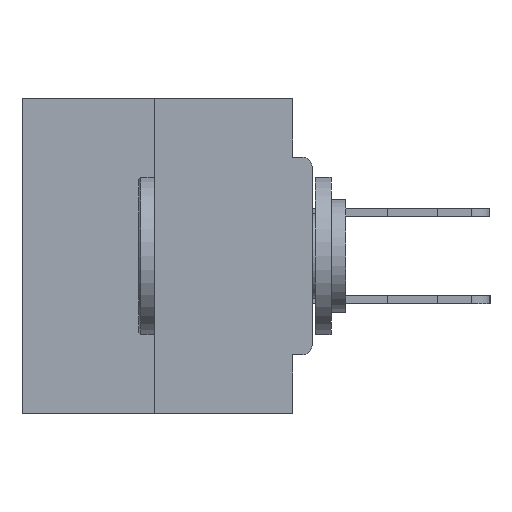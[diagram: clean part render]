
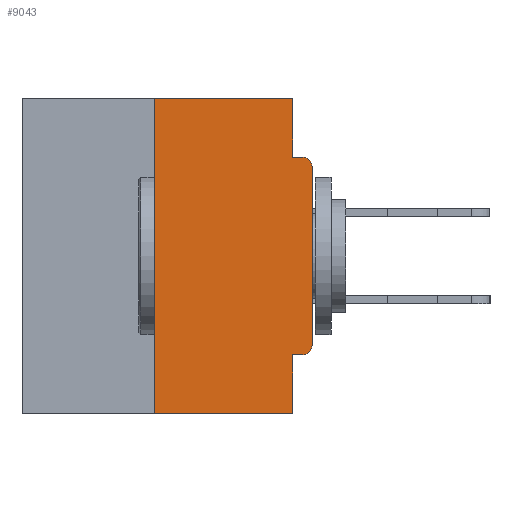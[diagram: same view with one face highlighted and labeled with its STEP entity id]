
A CAD part, left-side view. The second image highlights one B-rep face of the part: STEP entity #9043.
In plain terms, the highlighted planar face has unit normal (-1, 0, 0).
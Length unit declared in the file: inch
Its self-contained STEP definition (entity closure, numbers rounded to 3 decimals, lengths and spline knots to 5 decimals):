
#527 = CARTESIAN_POINT ( 'NONE',  ( 0., 0., -0.0935 ) ) ;
#830 = VECTOR ( 'NONE', #32874, 39.37008 ) ;
#1498 = CARTESIAN_POINT ( 'NONE',  ( 0., 0., 0. ) ) ;
#2949 = LINE ( 'NONE', #16704, #18603 ) ;
#3175 = LINE ( 'NONE', #33150, #6227 ) ;
#3206 = ORIENTED_EDGE ( 'NONE', *, *, #18143, .T. ) ;
#3600 = EDGE_CURVE ( 'NONE', #32147, #38464, #3175, .T. ) ;
#3841 = VERTEX_POINT ( 'NONE', #30647 ) ;
#5326 = LINE ( 'NONE', #1498, #29543 ) ;
#6178 = EDGE_CURVE ( 'NONE', #37746, #3841, #2949, .T. ) ;
#6227 = VECTOR ( 'NONE', #13628, 39.37008 ) ;
#6425 = CARTESIAN_POINT ( 'NONE',  ( 0., 0.25, 0. ) ) ;
#6603 = ORIENTED_EDGE ( 'NONE', *, *, #18887, .T. ) ;
#6707 = VECTOR ( 'NONE', #35863, 39.37008 ) ;
#7351 = DIRECTION ( 'NONE',  ( 0., 1., 0. ) ) ;
#9043 = ADVANCED_FACE ( 'NONE', ( #31865 ), #21742, .F. ) ;
#9212 = DIRECTION ( 'NONE',  ( -1., 0., 0. ) ) ;
#9318 = VERTEX_POINT ( 'NONE', #10560 ) ;
#9726 = CARTESIAN_POINT ( 'NONE',  ( 0., 0.031, 0. ) ) ;
#10375 = VERTEX_POINT ( 'NONE', #37322 ) ;
#10560 = CARTESIAN_POINT ( 'NONE',  ( 0., 0.015, -0.0935 ) ) ;
#11469 = AXIS2_PLACEMENT_3D ( 'NONE', #24979, #12421, #31970 ) ;
#12241 = EDGE_CURVE ( 'NONE', #3841, #30414, #36636, .T. ) ;
#12421 = DIRECTION ( 'NONE',  ( 1., 0., 0. ) ) ;
#12734 = CARTESIAN_POINT ( 'NONE',  ( 0., 0.031, -0.5 ) ) ;
#12976 = EDGE_CURVE ( 'NONE', #32429, #32147, #39574, .T. ) ;
#13628 = DIRECTION ( 'NONE',  ( 0., -1., 0. ) ) ;
#14148 = CIRCLE ( 'NONE', #14466, 0.015 ) ;
#14466 = AXIS2_PLACEMENT_3D ( 'NONE', #25701, #9212, #18907 ) ;
#14702 = CARTESIAN_POINT ( 'NONE',  ( 0., 0.25, 0. ) ) ;
#15215 = CIRCLE ( 'NONE', #40573, 0.015 ) ;
#16526 = DIRECTION ( 'NONE',  ( 0., -1., 0. ) ) ;
#16704 = CARTESIAN_POINT ( 'NONE',  ( 0., 0., -0.4065 ) ) ;
#17933 = VECTOR ( 'NONE', #29307, 39.37008 ) ;
#18143 = EDGE_CURVE ( 'NONE', #37746, #10375, #15215, .T. ) ;
#18603 = VECTOR ( 'NONE', #7351, 39.37008 ) ;
#18887 = EDGE_CURVE ( 'NONE', #32446, #9318, #14148, .T. ) ;
#18907 = DIRECTION ( 'NONE',  ( 0., 0., -1. ) ) ;
#18937 = ORIENTED_EDGE ( 'NONE', *, *, #34356, .T. ) ;
#19187 = ORIENTED_EDGE ( 'NONE', *, *, #12976, .F. ) ;
#19245 = DIRECTION ( 'NONE',  ( 0., 0., 1. ) ) ;
#19813 = VERTEX_POINT ( 'NONE', #25471 ) ;
#20963 = DIRECTION ( 'NONE',  ( 0., 0., 1. ) ) ;
#21742 = PLANE ( 'NONE',  #11469 ) ;
#21931 = ORIENTED_EDGE ( 'NONE', *, *, #32604, .T. ) ;
#22464 = EDGE_LOOP ( 'NONE', ( #37503, #19187, #18937, #27968, #35014, #3206, #21931, #6603, #24981, #36071 ) ) ;
#23118 = CARTESIAN_POINT ( 'NONE',  ( 0., 0.25, -0.5 ) ) ;
#24979 = CARTESIAN_POINT ( 'NONE',  ( 0., 0.46, 0. ) ) ;
#24981 = ORIENTED_EDGE ( 'NONE', *, *, #39985, .F. ) ;
#25471 = CARTESIAN_POINT ( 'NONE',  ( 0., 0.031, -0.0935 ) ) ;
#25658 = DIRECTION ( 'NONE',  ( 0., 0., -1. ) ) ;
#25701 = CARTESIAN_POINT ( 'NONE',  ( 0., 0.015, -0.1085 ) ) ;
#26360 = CARTESIAN_POINT ( 'NONE',  ( 0., 0., -0.1085 ) ) ;
#27088 = CARTESIAN_POINT ( 'NONE',  ( 0., 0.031, 0. ) ) ;
#27619 = VECTOR ( 'NONE', #16526, 39.37008 ) ;
#27968 = ORIENTED_EDGE ( 'NONE', *, *, #12241, .F. ) ;
#28331 = CARTESIAN_POINT ( 'NONE',  ( 0., 0.015, -0.3915 ) ) ;
#29307 = DIRECTION ( 'NONE',  ( 0., 0., -1. ) ) ;
#29543 = VECTOR ( 'NONE', #20963, 39.37008 ) ;
#30414 = VERTEX_POINT ( 'NONE', #12734 ) ;
#30647 = CARTESIAN_POINT ( 'NONE',  ( 0., 0.031, -0.4065 ) ) ;
#31421 = LINE ( 'NONE', #35448, #6707 ) ;
#31865 = FACE_OUTER_BOUND ( 'NONE', #22464, .T. ) ;
#31970 = DIRECTION ( 'NONE',  ( 0., 0., -1. ) ) ;
#32147 = VERTEX_POINT ( 'NONE', #14702 ) ;
#32266 = EDGE_CURVE ( 'NONE', #38464, #19813, #35034, .T. ) ;
#32429 = VERTEX_POINT ( 'NONE', #23118 ) ;
#32446 = VERTEX_POINT ( 'NONE', #26360 ) ;
#32604 = EDGE_CURVE ( 'NONE', #10375, #32446, #5326, .T. ) ;
#32874 = DIRECTION ( 'NONE',  ( 0., 0., -1. ) ) ;
#33150 = CARTESIAN_POINT ( 'NONE',  ( 0., 0.46, 0. ) ) ;
#34356 = EDGE_CURVE ( 'NONE', #32429, #30414, #31421, .T. ) ;
#35014 = ORIENTED_EDGE ( 'NONE', *, *, #6178, .F. ) ;
#35034 = LINE ( 'NONE', #9726, #17933 ) ;
#35148 = CARTESIAN_POINT ( 'NONE',  ( 0., 0.031, -0.5 ) ) ;
#35195 = DIRECTION ( 'NONE',  ( -1., 0., 0. ) ) ;
#35448 = CARTESIAN_POINT ( 'NONE',  ( 0., 0.46, -0.5 ) ) ;
#35685 = LINE ( 'NONE', #527, #27619 ) ;
#35863 = DIRECTION ( 'NONE',  ( 0., -1., 0. ) ) ;
#36071 = ORIENTED_EDGE ( 'NONE', *, *, #32266, .F. ) ;
#36636 = LINE ( 'NONE', #35148, #830 ) ;
#37322 = CARTESIAN_POINT ( 'NONE',  ( 0., 0., -0.3915 ) ) ;
#37503 = ORIENTED_EDGE ( 'NONE', *, *, #3600, .F. ) ;
#37746 = VERTEX_POINT ( 'NONE', #41497 ) ;
#38464 = VERTEX_POINT ( 'NONE', #27088 ) ;
#39104 = VECTOR ( 'NONE', #19245, 39.37008 ) ;
#39574 = LINE ( 'NONE', #6425, #39104 ) ;
#39985 = EDGE_CURVE ( 'NONE', #19813, #9318, #35685, .T. ) ;
#40573 = AXIS2_PLACEMENT_3D ( 'NONE', #28331, #35195, #25658 ) ;
#41497 = CARTESIAN_POINT ( 'NONE',  ( 0., 0.015, -0.4065 ) ) ;
